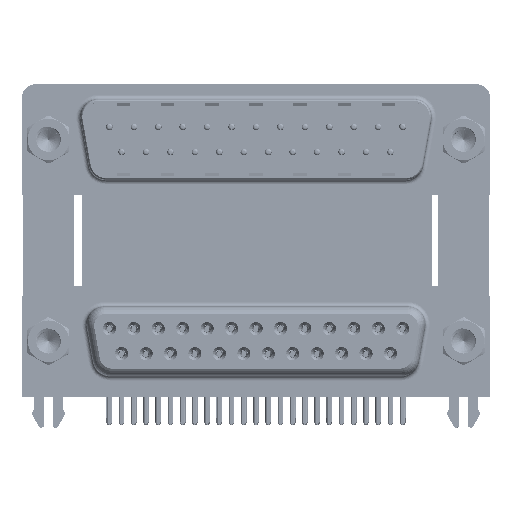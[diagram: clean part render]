
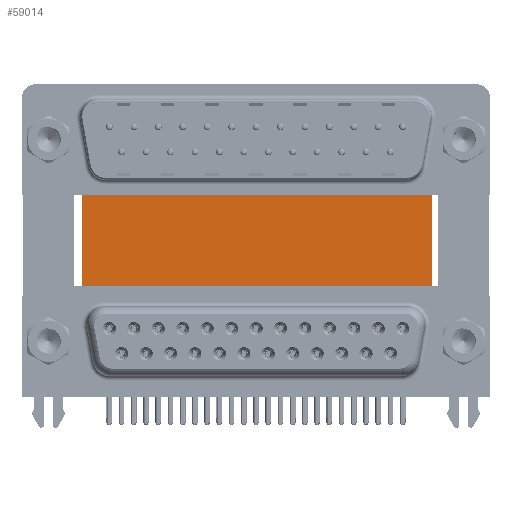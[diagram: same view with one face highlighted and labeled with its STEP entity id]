
A CAD part, top view. The second image highlights one B-rep face of the part: STEP entity #59014.
In plain terms, the highlighted planar face has unit normal (0, 0, 1).
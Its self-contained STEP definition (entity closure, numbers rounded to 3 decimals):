
#137 = EDGE_CURVE ( 'NONE', #54108, #37700, #37369, .T. ) ;
#459 = ORIENTED_EDGE ( 'NONE', *, *, #137, .F. ) ;
#1981 = EDGE_LOOP ( 'NONE', ( #12921, #459, #59384, #21103 ) ) ;
#3711 = CARTESIAN_POINT ( 'NONE',  ( 3.79, 16.585, -12. ) ) ;
#3821 = VECTOR ( 'NONE', #41148, 1000. ) ;
#4037 = CARTESIAN_POINT ( 'NONE',  ( 3.79, -3.735, -12. ) ) ;
#6547 = LINE ( 'NONE', #20850, #53423 ) ;
#10070 = VECTOR ( 'NONE', #40701, 1000. ) ;
#12921 = ORIENTED_EDGE ( 'NONE', *, *, #26676, .T. ) ;
#15760 = CARTESIAN_POINT ( 'NONE',  ( 3.79, 16.585, -12. ) ) ;
#19921 = AXIS2_PLACEMENT_3D ( 'NONE', #3711, #45457, #21756 ) ;
#20134 = DIRECTION ( 'NONE',  ( 1., 0., 0. ) ) ;
#20850 = CARTESIAN_POINT ( 'NONE',  ( 3.79, -3.735, -12. ) ) ;
#21103 = ORIENTED_EDGE ( 'NONE', *, *, #58468, .T. ) ;
#21672 = CARTESIAN_POINT ( 'NONE',  ( 3.79, 16.585, -12. ) ) ;
#21756 = DIRECTION ( 'NONE',  ( -1., 0., 0. ) ) ;
#24295 = VECTOR ( 'NONE', #20134, 1000. ) ;
#26676 = EDGE_CURVE ( 'NONE', #35589, #37700, #6547, .T. ) ;
#31114 = CARTESIAN_POINT ( 'NONE',  ( 3.79, 16.585, -12. ) ) ;
#32323 = PLANE ( 'NONE',  #19921 ) ;
#33905 = VERTEX_POINT ( 'NONE', #31114 ) ;
#35589 = VERTEX_POINT ( 'NONE', #4037 ) ;
#37001 = FACE_OUTER_BOUND ( 'NONE', #1981, .T. ) ;
#37369 = LINE ( 'NONE', #40843, #3821 ) ;
#37700 = VERTEX_POINT ( 'NONE', #38743 ) ;
#38743 = CARTESIAN_POINT ( 'NONE',  ( 43.43, -3.735, -12. ) ) ;
#39530 = CARTESIAN_POINT ( 'NONE',  ( 43.43, 16.585, -12. ) ) ;
#40701 = DIRECTION ( 'NONE',  ( 0., -1., 0. ) ) ;
#40785 = DIRECTION ( 'NONE',  ( 1., 0., 0. ) ) ;
#40843 = CARTESIAN_POINT ( 'NONE',  ( 43.43, 16.585, -12. ) ) ;
#41148 = DIRECTION ( 'NONE',  ( 0., -1., 0. ) ) ;
#42908 = EDGE_CURVE ( 'NONE', #33905, #54108, #43843, .T. ) ;
#43843 = LINE ( 'NONE', #15760, #24295 ) ;
#45457 = DIRECTION ( 'NONE',  ( 0., 0., -1. ) ) ;
#53423 = VECTOR ( 'NONE', #40785, 1000. ) ;
#54108 = VERTEX_POINT ( 'NONE', #39530 ) ;
#58468 = EDGE_CURVE ( 'NONE', #33905, #35589, #60034, .T. ) ;
#59014 = ADVANCED_FACE ( 'NONE', ( #37001 ), #32323, .F. ) ;
#59384 = ORIENTED_EDGE ( 'NONE', *, *, #42908, .F. ) ;
#60034 = LINE ( 'NONE', #21672, #10070 ) ;
